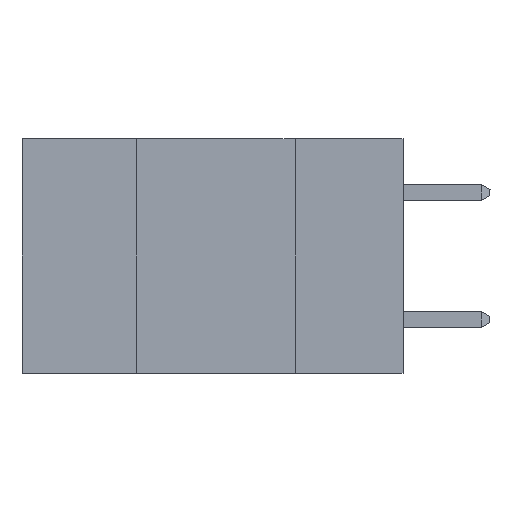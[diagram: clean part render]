
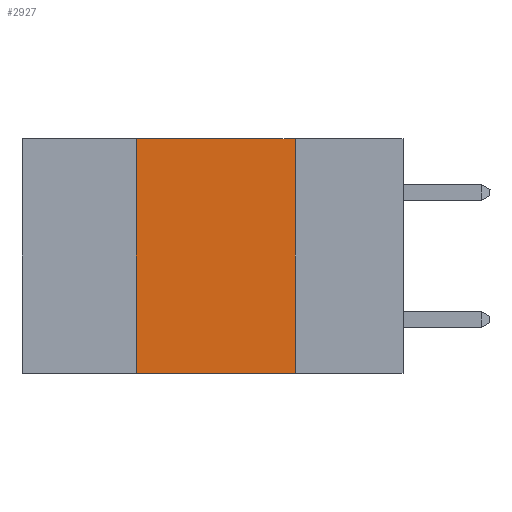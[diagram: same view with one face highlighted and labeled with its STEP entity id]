
A CAD part, left-side view. The second image highlights one B-rep face of the part: STEP entity #2927.
In plain terms, the highlighted planar face has unit normal (-1, 0, 0).
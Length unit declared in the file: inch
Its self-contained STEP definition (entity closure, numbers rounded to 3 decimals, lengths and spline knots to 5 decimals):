
#178 = CARTESIAN_POINT ( 'NONE',  ( 0., 0.6, 0. ) ) ;
#279 = ORIENTED_EDGE ( 'NONE', *, *, #10162, .T. ) ;
#884 = DIRECTION ( 'NONE',  ( 1., 0., 0. ) ) ;
#1056 = DIRECTION ( 'NONE',  ( 0., 0., 1. ) ) ;
#1690 = LINE ( 'NONE', #1949, #5888 ) ;
#1949 = CARTESIAN_POINT ( 'NONE',  ( 0., 0.17, 0. ) ) ;
#2927 = ADVANCED_FACE ( 'NONE', ( #9394 ), #22334, .F. ) ;
#3145 = CARTESIAN_POINT ( 'NONE',  ( 0., 0.42, 0. ) ) ;
#4535 = CARTESIAN_POINT ( 'NONE',  ( 0., 0.17, -0.37 ) ) ;
#4772 = DIRECTION ( 'NONE',  ( 0., -1., 0. ) ) ;
#5032 = VERTEX_POINT ( 'NONE', #16345 ) ;
#5291 = ORIENTED_EDGE ( 'NONE', *, *, #16265, .F. ) ;
#5552 = LINE ( 'NONE', #14616, #10614 ) ;
#5854 = VERTEX_POINT ( 'NONE', #11911 ) ;
#5888 = VECTOR ( 'NONE', #27074, 39.37008 ) ;
#7183 = EDGE_CURVE ( 'NONE', #5854, #11539, #1690, .T. ) ;
#7966 = CARTESIAN_POINT ( 'NONE',  ( 0., 0.42, 0. ) ) ;
#9394 = FACE_OUTER_BOUND ( 'NONE', #19593, .T. ) ;
#9910 = ORIENTED_EDGE ( 'NONE', *, *, #16577, .F. ) ;
#10033 = VECTOR ( 'NONE', #1056, 39.37008 ) ;
#10162 = EDGE_CURVE ( 'NONE', #5032, #11539, #5552, .T. ) ;
#10614 = VECTOR ( 'NONE', #18984, 39.37008 ) ;
#11539 = VERTEX_POINT ( 'NONE', #4535 ) ;
#11911 = CARTESIAN_POINT ( 'NONE',  ( 0., 0.17, 0. ) ) ;
#14616 = CARTESIAN_POINT ( 'NONE',  ( 0., 0.6, -0.37 ) ) ;
#15433 = CARTESIAN_POINT ( 'NONE',  ( 0., 0.6, 0. ) ) ;
#16265 = EDGE_CURVE ( 'NONE', #5032, #27691, #24313, .T. ) ;
#16315 = VECTOR ( 'NONE', #4772, 39.37008 ) ;
#16345 = CARTESIAN_POINT ( 'NONE',  ( 0., 0.42, -0.37 ) ) ;
#16577 = EDGE_CURVE ( 'NONE', #27691, #5854, #23582, .T. ) ;
#18984 = DIRECTION ( 'NONE',  ( 0., -1., 0. ) ) ;
#19518 = AXIS2_PLACEMENT_3D ( 'NONE', #15433, #884, #24278 ) ;
#19593 = EDGE_LOOP ( 'NONE', ( #27311, #9910, #5291, #279 ) ) ;
#22334 = PLANE ( 'NONE',  #19518 ) ;
#23582 = LINE ( 'NONE', #178, #16315 ) ;
#24278 = DIRECTION ( 'NONE',  ( 0., 0., -1. ) ) ;
#24313 = LINE ( 'NONE', #3145, #10033 ) ;
#27074 = DIRECTION ( 'NONE',  ( 0., 0., -1. ) ) ;
#27311 = ORIENTED_EDGE ( 'NONE', *, *, #7183, .F. ) ;
#27691 = VERTEX_POINT ( 'NONE', #7966 ) ;
